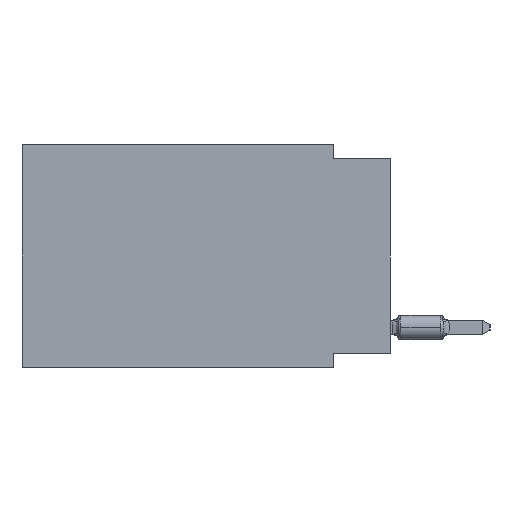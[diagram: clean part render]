
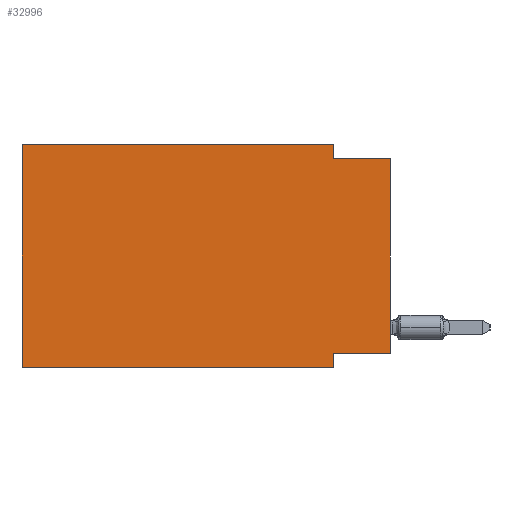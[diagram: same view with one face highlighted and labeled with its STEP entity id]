
A CAD part, left-side view. The second image highlights one B-rep face of the part: STEP entity #32996.
In plain terms, the highlighted planar face has unit normal (-1, 0, 0).
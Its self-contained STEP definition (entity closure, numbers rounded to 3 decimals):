
#525 = VERTEX_POINT ( 'NONE', #33015 ) ;
#606 = LINE ( 'NONE', #21650, #1132 ) ;
#670 = DIRECTION ( 'NONE',  ( 0., 0., 1. ) ) ;
#1116 = ORIENTED_EDGE ( 'NONE', *, *, #29912, .T. ) ;
#1132 = VECTOR ( 'NONE', #32543, 1000. ) ;
#1743 = ORIENTED_EDGE ( 'NONE', *, *, #2719, .F. ) ;
#1868 = CARTESIAN_POINT ( 'NONE',  ( 0., 16.383, 0. ) ) ;
#2215 = DIRECTION ( 'NONE',  ( 0., -1., 0. ) ) ;
#2614 = VECTOR ( 'NONE', #27347, 1000. ) ;
#2719 = EDGE_CURVE ( 'NONE', #28735, #21580, #606, .T. ) ;
#3383 = EDGE_CURVE ( 'NONE', #28735, #20368, #26163, .T. ) ;
#3806 = VECTOR ( 'NONE', #7536, 1000. ) ;
#4765 = ORIENTED_EDGE ( 'NONE', *, *, #14947, .F. ) ;
#5696 = DIRECTION ( 'NONE',  ( 0., -1., 0. ) ) ;
#5855 = AXIS2_PLACEMENT_3D ( 'NONE', #28532, #14830, #20617 ) ;
#6002 = CARTESIAN_POINT ( 'NONE',  ( 0., 0., -0.635 ) ) ;
#6074 = CARTESIAN_POINT ( 'NONE',  ( 0., 2.54, 0. ) ) ;
#7084 = CARTESIAN_POINT ( 'NONE',  ( 0., 2.54, -0.635 ) ) ;
#7536 = DIRECTION ( 'NONE',  ( 0., 0., 1. ) ) ;
#7553 = VECTOR ( 'NONE', #21719, 1000. ) ;
#9196 = LINE ( 'NONE', #17279, #2614 ) ;
#9531 = ORIENTED_EDGE ( 'NONE', *, *, #31591, .F. ) ;
#10246 = PLANE ( 'NONE',  #5855 ) ;
#10424 = VECTOR ( 'NONE', #2215, 1000. ) ;
#12431 = ORIENTED_EDGE ( 'NONE', *, *, #3383, .T. ) ;
#12975 = VERTEX_POINT ( 'NONE', #1868 ) ;
#13606 = DIRECTION ( 'NONE',  ( 0., 0., -1. ) ) ;
#13993 = CARTESIAN_POINT ( 'NONE',  ( 0., 0., 0. ) ) ;
#14830 = DIRECTION ( 'NONE',  ( 1., 0., 0. ) ) ;
#14947 = EDGE_CURVE ( 'NONE', #26809, #20368, #15535, .T. ) ;
#15535 = LINE ( 'NONE', #18354, #10424 ) ;
#16411 = LINE ( 'NONE', #6074, #31575 ) ;
#17065 = ORIENTED_EDGE ( 'NONE', *, *, #28650, .F. ) ;
#17279 = CARTESIAN_POINT ( 'NONE',  ( 0., 16.383, -9.906 ) ) ;
#18054 = CARTESIAN_POINT ( 'NONE',  ( 0., 16.383, 0. ) ) ;
#18354 = CARTESIAN_POINT ( 'NONE',  ( 0., 0., -0.635 ) ) ;
#20368 = VERTEX_POINT ( 'NONE', #6002 ) ;
#20617 = DIRECTION ( 'NONE',  ( 0., 0., -1. ) ) ;
#21512 = CARTESIAN_POINT ( 'NONE',  ( 0., 2.54, -9.906 ) ) ;
#21580 = VERTEX_POINT ( 'NONE', #30464 ) ;
#21650 = CARTESIAN_POINT ( 'NONE',  ( 0., 0., -9.271 ) ) ;
#21719 = DIRECTION ( 'NONE',  ( 0., 0., -1. ) ) ;
#23258 = ORIENTED_EDGE ( 'NONE', *, *, #23501, .F. ) ;
#23501 = EDGE_CURVE ( 'NONE', #525, #12975, #31402, .T. ) ;
#23687 = LINE ( 'NONE', #27340, #7553 ) ;
#24271 = EDGE_LOOP ( 'NONE', ( #12431, #4765, #9531, #17065, #23258, #1116, #25697, #1743 ) ) ;
#24822 = CARTESIAN_POINT ( 'NONE',  ( 0., 0., -9.271 ) ) ;
#24975 = VECTOR ( 'NONE', #5696, 1000. ) ;
#25697 = ORIENTED_EDGE ( 'NONE', *, *, #26013, .F. ) ;
#25701 = VERTEX_POINT ( 'NONE', #30248 ) ;
#26013 = EDGE_CURVE ( 'NONE', #21580, #34107, #23687, .T. ) ;
#26163 = LINE ( 'NONE', #13993, #29175 ) ;
#26809 = VERTEX_POINT ( 'NONE', #7084 ) ;
#27340 = CARTESIAN_POINT ( 'NONE',  ( 0., 2.54, -9.906 ) ) ;
#27347 = DIRECTION ( 'NONE',  ( 0., -1., 0. ) ) ;
#28532 = CARTESIAN_POINT ( 'NONE',  ( 0., 16.383, 0. ) ) ;
#28650 = EDGE_CURVE ( 'NONE', #12975, #25701, #29743, .T. ) ;
#28735 = VERTEX_POINT ( 'NONE', #24822 ) ;
#29175 = VECTOR ( 'NONE', #670, 1000. ) ;
#29743 = LINE ( 'NONE', #32555, #24975 ) ;
#29912 = EDGE_CURVE ( 'NONE', #525, #34107, #9196, .T. ) ;
#30248 = CARTESIAN_POINT ( 'NONE',  ( 0., 2.54, 0. ) ) ;
#30464 = CARTESIAN_POINT ( 'NONE',  ( 0., 2.54, -9.271 ) ) ;
#31402 = LINE ( 'NONE', #18054, #3806 ) ;
#31575 = VECTOR ( 'NONE', #13606, 1000. ) ;
#31591 = EDGE_CURVE ( 'NONE', #25701, #26809, #16411, .T. ) ;
#32543 = DIRECTION ( 'NONE',  ( 0., 1., 0. ) ) ;
#32555 = CARTESIAN_POINT ( 'NONE',  ( 0., 16.383, 0. ) ) ;
#32946 = FACE_OUTER_BOUND ( 'NONE', #24271, .T. ) ;
#32996 = ADVANCED_FACE ( 'NONE', ( #32946 ), #10246, .F. ) ;
#33015 = CARTESIAN_POINT ( 'NONE',  ( 0., 16.383, -9.906 ) ) ;
#34107 = VERTEX_POINT ( 'NONE', #21512 ) ;
